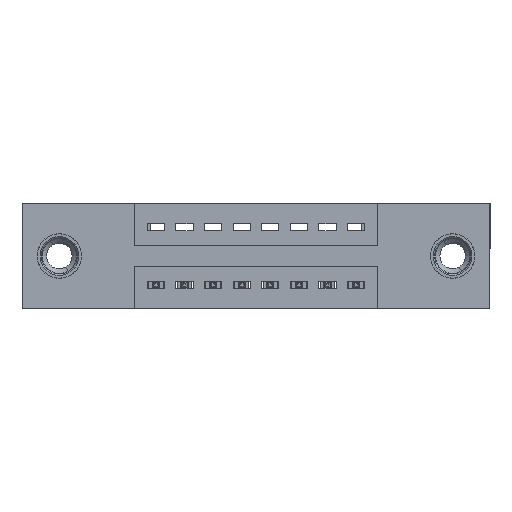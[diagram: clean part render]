
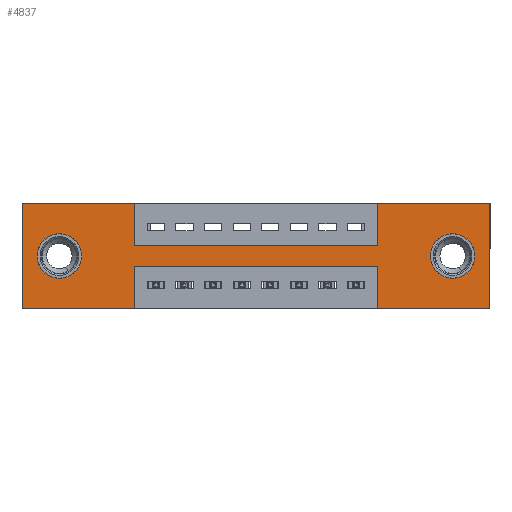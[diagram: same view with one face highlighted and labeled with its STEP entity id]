
A CAD part, front view. The second image highlights one B-rep face of the part: STEP entity #4837.
In plain terms, the highlighted planar face has unit normal (0, -1, 0).
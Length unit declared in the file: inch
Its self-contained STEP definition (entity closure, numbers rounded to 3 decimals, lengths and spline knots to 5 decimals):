
#5 = CARTESIAN_POINT ( 'NONE',  ( 0.3925, 0., -0.22 ) ) ;
#756 = VERTEX_POINT ( 'NONE', #6746 ) ;
#773 = ORIENTED_EDGE ( 'NONE', *, *, #4743, .T. ) ;
#824 = LINE ( 'NONE', #9165, #1968 ) ;
#830 = LINE ( 'NONE', #5408, #9624 ) ;
#928 = VERTEX_POINT ( 'NONE', #4916 ) ;
#965 = DIRECTION ( 'NONE',  ( 0., 0., -1. ) ) ;
#1038 = CARTESIAN_POINT ( 'NONE',  ( 0.13, 0., -0.107 ) ) ;
#1123 = VERTEX_POINT ( 'NONE', #13847 ) ;
#1293 = VERTEX_POINT ( 'NONE', #10938 ) ;
#1379 = DIRECTION ( 'NONE',  ( 0., 0., -1. ) ) ;
#1407 = EDGE_CURVE ( 'NONE', #2458, #4723, #10197, .T. ) ;
#1608 = ORIENTED_EDGE ( 'NONE', *, *, #8654, .F. ) ;
#1643 = CARTESIAN_POINT ( 'NONE',  ( 0.3925, 0., -0.22 ) ) ;
#1660 = ORIENTED_EDGE ( 'NONE', *, *, #12517, .F. ) ;
#1725 = DIRECTION ( 'NONE',  ( -1., 0., 0. ) ) ;
#1809 = FACE_OUTER_BOUND ( 'NONE', #5849, .T. ) ;
#1842 = CARTESIAN_POINT ( 'NONE',  ( 0., 0., 0. ) ) ;
#1904 = CARTESIAN_POINT ( 'NONE',  ( 1.2425, 0., 0. ) ) ;
#1915 = LINE ( 'NONE', #4322, #5107 ) ;
#1954 = CIRCLE ( 'NONE', #3438, 0.078 ) ;
#1968 = VECTOR ( 'NONE', #6899, 39.37008 ) ;
#1987 = ORIENTED_EDGE ( 'NONE', *, *, #2323, .F. ) ;
#2020 = ORIENTED_EDGE ( 'NONE', *, *, #5607, .F. ) ;
#2203 = AXIS2_PLACEMENT_3D ( 'NONE', #8834, #13603, #8614 ) ;
#2301 = CARTESIAN_POINT ( 'NONE',  ( 0., 0., 0. ) ) ;
#2323 = EDGE_CURVE ( 'NONE', #4723, #4947, #9121, .T. ) ;
#2404 = ORIENTED_EDGE ( 'NONE', *, *, #2787, .T. ) ;
#2458 = VERTEX_POINT ( 'NONE', #15122 ) ;
#2787 = EDGE_CURVE ( 'NONE', #13552, #10761, #13748, .T. ) ;
#2904 = DIRECTION ( 'NONE',  ( 0., -1., 0. ) ) ;
#2965 = VECTOR ( 'NONE', #12514, 39.37008 ) ;
#3079 = LINE ( 'NONE', #1904, #5166 ) ;
#3098 = AXIS2_PLACEMENT_3D ( 'NONE', #8491, #9805, #1379 ) ;
#3141 = FACE_BOUND ( 'NONE', #5988, .T. ) ;
#3190 = DIRECTION ( 'NONE',  ( 0., 0., -1. ) ) ;
#3438 = AXIS2_PLACEMENT_3D ( 'NONE', #14504, #7389, #8571 ) ;
#3521 = ORIENTED_EDGE ( 'NONE', *, *, #8304, .F. ) ;
#3629 = CARTESIAN_POINT ( 'NONE',  ( 1.635, 0., 0. ) ) ;
#3832 = CARTESIAN_POINT ( 'NONE',  ( 0.3925, 0., 0. ) ) ;
#4060 = DIRECTION ( 'NONE',  ( 0., 0., -1. ) ) ;
#4070 = CARTESIAN_POINT ( 'NONE',  ( 0., 0., 0. ) ) ;
#4167 = ORIENTED_EDGE ( 'NONE', *, *, #12985, .T. ) ;
#4220 = PLANE ( 'NONE',  #13816 ) ;
#4322 = CARTESIAN_POINT ( 'NONE',  ( 0.3925, 0., -0.15 ) ) ;
#4723 = VERTEX_POINT ( 'NONE', #3629 ) ;
#4743 = EDGE_CURVE ( 'NONE', #10761, #13552, #15069, .T. ) ;
#4754 = CARTESIAN_POINT ( 'NONE',  ( 1.635, 0., -0.37 ) ) ;
#4831 = CARTESIAN_POINT ( 'NONE',  ( 1.505, 0., -0.185 ) ) ;
#4837 = ADVANCED_FACE ( 'NONE', ( #3141, #6484, #1809 ), #4220, .T. ) ;
#4916 = CARTESIAN_POINT ( 'NONE',  ( 0., 0., -0.37 ) ) ;
#4947 = VERTEX_POINT ( 'NONE', #4754 ) ;
#5006 = ORIENTED_EDGE ( 'NONE', *, *, #8319, .F. ) ;
#5107 = VECTOR ( 'NONE', #6907, 39.37008 ) ;
#5166 = VECTOR ( 'NONE', #10347, 39.37008 ) ;
#5408 = CARTESIAN_POINT ( 'NONE',  ( 0., 0., -0.37 ) ) ;
#5607 = EDGE_CURVE ( 'NONE', #6234, #14925, #14769, .T. ) ;
#5849 = EDGE_LOOP ( 'NONE', ( #13714, #2020, #7698, #5006, #1987, #9735, #1660, #3521, #11353, #10616, #1608, #14653 ) ) ;
#5939 = VERTEX_POINT ( 'NONE', #12365 ) ;
#5988 = EDGE_LOOP ( 'NONE', ( #773, #2404 ) ) ;
#6134 = LINE ( 'NONE', #12255, #10062 ) ;
#6234 = VERTEX_POINT ( 'NONE', #11494 ) ;
#6388 = EDGE_CURVE ( 'NONE', #14925, #1293, #6134, .T. ) ;
#6397 = LINE ( 'NONE', #3832, #13917 ) ;
#6484 = FACE_BOUND ( 'NONE', #9590, .T. ) ;
#6552 = DIRECTION ( 'NONE',  ( 0., 0., -1. ) ) ;
#6746 = CARTESIAN_POINT ( 'NONE',  ( 1.2425, 0., -0.37 ) ) ;
#6899 = DIRECTION ( 'NONE',  ( 0., 0., 1. ) ) ;
#6907 = DIRECTION ( 'NONE',  ( 1., 0., 0. ) ) ;
#7389 = DIRECTION ( 'NONE',  ( 0., 1., 0. ) ) ;
#7434 = LINE ( 'NONE', #7595, #2965 ) ;
#7595 = CARTESIAN_POINT ( 'NONE',  ( 0., 0., 0. ) ) ;
#7698 = ORIENTED_EDGE ( 'NONE', *, *, #13554, .F. ) ;
#7699 = ORIENTED_EDGE ( 'NONE', *, *, #12800, .T. ) ;
#7857 = VECTOR ( 'NONE', #1725, 39.37008 ) ;
#8019 = DIRECTION ( 'NONE',  ( -1., 0., 0. ) ) ;
#8304 = EDGE_CURVE ( 'NONE', #1123, #14651, #1915, .T. ) ;
#8319 = EDGE_CURVE ( 'NONE', #4947, #756, #830, .T. ) ;
#8491 = CARTESIAN_POINT ( 'NONE',  ( 1.505, 0., -0.185 ) ) ;
#8571 = DIRECTION ( 'NONE',  ( 0., 0., 1. ) ) ;
#8581 = DIRECTION ( 'NONE',  ( 0., 0., -1. ) ) ;
#8614 = DIRECTION ( 'NONE',  ( 0., 0., 1. ) ) ;
#8627 = VECTOR ( 'NONE', #14550, 39.37008 ) ;
#8654 = EDGE_CURVE ( 'NONE', #928, #12627, #10021, .T. ) ;
#8767 = CARTESIAN_POINT ( 'NONE',  ( 0.3925, 0., 0. ) ) ;
#8834 = CARTESIAN_POINT ( 'NONE',  ( 0.13, 0., -0.185 ) ) ;
#9121 = LINE ( 'NONE', #13894, #9214 ) ;
#9165 = CARTESIAN_POINT ( 'NONE',  ( 1.2425, 0., -0.37 ) ) ;
#9214 = VECTOR ( 'NONE', #3190, 39.37008 ) ;
#9590 = EDGE_LOOP ( 'NONE', ( #7699, #4167 ) ) ;
#9624 = VECTOR ( 'NONE', #8019, 39.37008 ) ;
#9684 = AXIS2_PLACEMENT_3D ( 'NONE', #4831, #10794, #965 ) ;
#9735 = ORIENTED_EDGE ( 'NONE', *, *, #1407, .F. ) ;
#9766 = CARTESIAN_POINT ( 'NONE',  ( 0., 0., -0.37 ) ) ;
#9805 = DIRECTION ( 'NONE',  ( 0., 1., 0. ) ) ;
#10021 = LINE ( 'NONE', #4070, #8627 ) ;
#10062 = VECTOR ( 'NONE', #8581, 39.37008 ) ;
#10197 = LINE ( 'NONE', #1842, #14405 ) ;
#10347 = DIRECTION ( 'NONE',  ( 0., 0., 1. ) ) ;
#10616 = ORIENTED_EDGE ( 'NONE', *, *, #13820, .F. ) ;
#10761 = VERTEX_POINT ( 'NONE', #11312 ) ;
#10794 = DIRECTION ( 'NONE',  ( 0., 1., 0. ) ) ;
#10938 = CARTESIAN_POINT ( 'NONE',  ( 0.3925, 0., -0.37 ) ) ;
#11312 = CARTESIAN_POINT ( 'NONE',  ( 1.505, 0., -0.107 ) ) ;
#11353 = ORIENTED_EDGE ( 'NONE', *, *, #12790, .F. ) ;
#11461 = DIRECTION ( 'NONE',  ( 1., 0., 0. ) ) ;
#11494 = CARTESIAN_POINT ( 'NONE',  ( 1.2425, 0., -0.22 ) ) ;
#11861 = CARTESIAN_POINT ( 'NONE',  ( 1.2425, 0., -0.15 ) ) ;
#12255 = CARTESIAN_POINT ( 'NONE',  ( 0.3925, 0., -0.37 ) ) ;
#12365 = CARTESIAN_POINT ( 'NONE',  ( 0.13, 0., -0.263 ) ) ;
#12475 = VECTOR ( 'NONE', #13434, 39.37008 ) ;
#12514 = DIRECTION ( 'NONE',  ( 1., 0., 0. ) ) ;
#12517 = EDGE_CURVE ( 'NONE', #14651, #2458, #3079, .T. ) ;
#12627 = VERTEX_POINT ( 'NONE', #2301 ) ;
#12767 = VERTEX_POINT ( 'NONE', #8767 ) ;
#12790 = EDGE_CURVE ( 'NONE', #12767, #1123, #6397, .T. ) ;
#12800 = EDGE_CURVE ( 'NONE', #14118, #5939, #12928, .T. ) ;
#12928 = CIRCLE ( 'NONE', #2203, 0.078 ) ;
#12985 = EDGE_CURVE ( 'NONE', #5939, #14118, #1954, .T. ) ;
#13434 = DIRECTION ( 'NONE',  ( -1., 0., 0. ) ) ;
#13552 = VERTEX_POINT ( 'NONE', #14166 ) ;
#13554 = EDGE_CURVE ( 'NONE', #756, #6234, #824, .T. ) ;
#13603 = DIRECTION ( 'NONE',  ( 0., 1., 0. ) ) ;
#13714 = ORIENTED_EDGE ( 'NONE', *, *, #6388, .F. ) ;
#13748 = CIRCLE ( 'NONE', #9684, 0.078 ) ;
#13816 = AXIS2_PLACEMENT_3D ( 'NONE', #13841, #2904, #6552 ) ;
#13820 = EDGE_CURVE ( 'NONE', #12627, #12767, #7434, .T. ) ;
#13841 = CARTESIAN_POINT ( 'NONE',  ( 0., 0., -0.37 ) ) ;
#13847 = CARTESIAN_POINT ( 'NONE',  ( 0.3925, 0., -0.15 ) ) ;
#13894 = CARTESIAN_POINT ( 'NONE',  ( 1.635, 0., 0. ) ) ;
#13917 = VECTOR ( 'NONE', #4060, 39.37008 ) ;
#14118 = VERTEX_POINT ( 'NONE', #1038 ) ;
#14166 = CARTESIAN_POINT ( 'NONE',  ( 1.505, 0., -0.263 ) ) ;
#14405 = VECTOR ( 'NONE', #11461, 39.37008 ) ;
#14504 = CARTESIAN_POINT ( 'NONE',  ( 0.13, 0., -0.185 ) ) ;
#14529 = LINE ( 'NONE', #9766, #12475 ) ;
#14550 = DIRECTION ( 'NONE',  ( 0., 0., 1. ) ) ;
#14651 = VERTEX_POINT ( 'NONE', #11861 ) ;
#14653 = ORIENTED_EDGE ( 'NONE', *, *, #15111, .F. ) ;
#14769 = LINE ( 'NONE', #1643, #7857 ) ;
#14925 = VERTEX_POINT ( 'NONE', #5 ) ;
#15069 = CIRCLE ( 'NONE', #3098, 0.078 ) ;
#15111 = EDGE_CURVE ( 'NONE', #1293, #928, #14529, .T. ) ;
#15122 = CARTESIAN_POINT ( 'NONE',  ( 1.2425, 0., 0. ) ) ;
